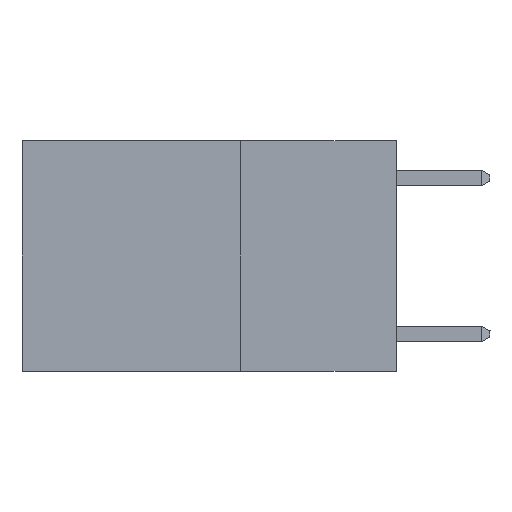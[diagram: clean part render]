
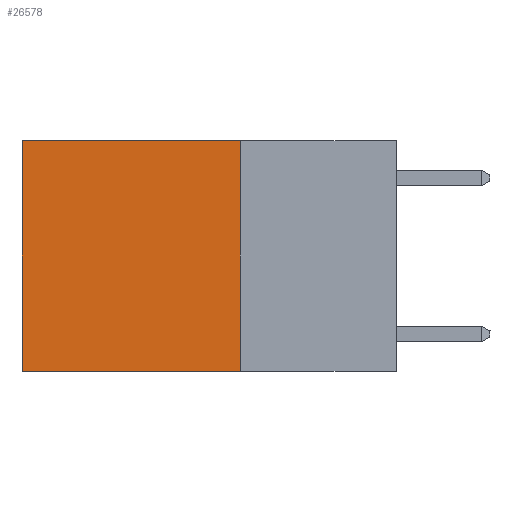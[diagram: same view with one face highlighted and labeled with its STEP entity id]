
A CAD part, left-side view. The second image highlights one B-rep face of the part: STEP entity #26578.
In plain terms, the highlighted planar face has unit normal (-1, 0, 0).
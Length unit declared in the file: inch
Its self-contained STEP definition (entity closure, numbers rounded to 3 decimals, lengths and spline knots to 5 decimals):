
#968 = CARTESIAN_POINT ( 'NONE',  ( 0.2625, 0.25, 0. ) ) ;
#1466 = CARTESIAN_POINT ( 'NONE',  ( 0.2625, 0.6, -0.37 ) ) ;
#1827 = CARTESIAN_POINT ( 'NONE',  ( 0.2625, 0.25, -0.37 ) ) ;
#1937 = VERTEX_POINT ( 'NONE', #1827 ) ;
#2049 = DIRECTION ( 'NONE',  ( 0., 1., 0. ) ) ;
#2165 = AXIS2_PLACEMENT_3D ( 'NONE', #16266, #6799, #23160 ) ;
#3903 = EDGE_CURVE ( 'NONE', #12796, #1937, #16141, .T. ) ;
#4387 = CARTESIAN_POINT ( 'NONE',  ( 0.2625, 0.25, 0. ) ) ;
#4939 = ORIENTED_EDGE ( 'NONE', *, *, #19382, .T. ) ;
#5259 = ORIENTED_EDGE ( 'NONE', *, *, #19637, .T. ) ;
#6799 = DIRECTION ( 'NONE',  ( 1., 0., 0. ) ) ;
#9393 = ORIENTED_EDGE ( 'NONE', *, *, #3903, .F. ) ;
#9397 = VERTEX_POINT ( 'NONE', #15179 ) ;
#10946 = VECTOR ( 'NONE', #2049, 39.37008 ) ;
#12774 = LINE ( 'NONE', #968, #18244 ) ;
#12796 = VERTEX_POINT ( 'NONE', #4387 ) ;
#14372 = DIRECTION ( 'NONE',  ( 0., 0., -1. ) ) ;
#14410 = EDGE_LOOP ( 'NONE', ( #4939, #26342, #9393, #5259 ) ) ;
#15179 = CARTESIAN_POINT ( 'NONE',  ( 0.2625, 0.6, 0. ) ) ;
#16141 = LINE ( 'NONE', #22760, #27478 ) ;
#16266 = CARTESIAN_POINT ( 'NONE',  ( 0.2625, 0.25, 0. ) ) ;
#17796 = CARTESIAN_POINT ( 'NONE',  ( 0.2625, 0.6, 0. ) ) ;
#18244 = VECTOR ( 'NONE', #19995, 39.37008 ) ;
#19382 = EDGE_CURVE ( 'NONE', #9397, #23849, #26045, .T. ) ;
#19637 = EDGE_CURVE ( 'NONE', #12796, #9397, #12774, .T. ) ;
#19995 = DIRECTION ( 'NONE',  ( 0., 1., 0. ) ) ;
#20802 = VECTOR ( 'NONE', #14372, 39.37008 ) ;
#20934 = PLANE ( 'NONE',  #2165 ) ;
#22525 = LINE ( 'NONE', #27623, #10946 ) ;
#22760 = CARTESIAN_POINT ( 'NONE',  ( 0.2625, 0.25, 0. ) ) ;
#22766 = EDGE_CURVE ( 'NONE', #1937, #23849, #22525, .T. ) ;
#23160 = DIRECTION ( 'NONE',  ( 0., 0., -1. ) ) ;
#23849 = VERTEX_POINT ( 'NONE', #1466 ) ;
#25011 = DIRECTION ( 'NONE',  ( 0., 0., -1. ) ) ;
#26045 = LINE ( 'NONE', #17796, #20802 ) ;
#26342 = ORIENTED_EDGE ( 'NONE', *, *, #22766, .F. ) ;
#26578 = ADVANCED_FACE ( 'NONE', ( #28245 ), #20934, .F. ) ;
#27478 = VECTOR ( 'NONE', #25011, 39.37008 ) ;
#27623 = CARTESIAN_POINT ( 'NONE',  ( 0.2625, 0.25, -0.37 ) ) ;
#28245 = FACE_OUTER_BOUND ( 'NONE', #14410, .T. ) ;
